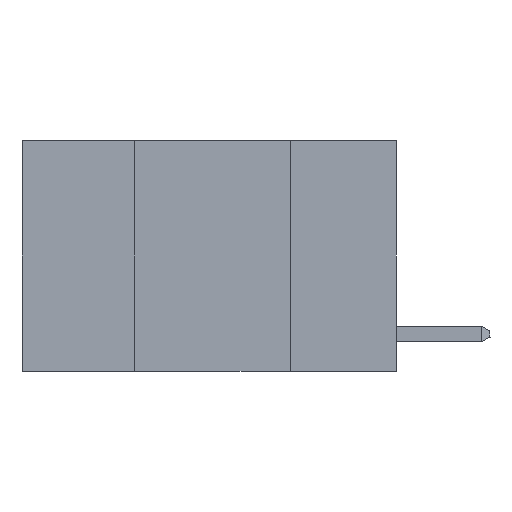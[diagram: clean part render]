
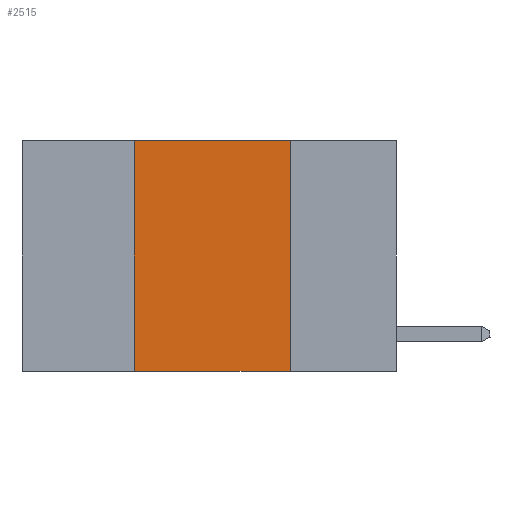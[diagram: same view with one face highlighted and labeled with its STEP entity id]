
A CAD part, left-side view. The second image highlights one B-rep face of the part: STEP entity #2515.
In plain terms, the highlighted planar face has unit normal (-1, 0, 0).
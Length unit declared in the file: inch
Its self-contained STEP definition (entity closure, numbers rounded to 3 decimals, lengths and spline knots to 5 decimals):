
#489 = DIRECTION ( 'NONE',  ( 1., 0., 0. ) ) ;
#502 = DIRECTION ( 'NONE',  ( 0., -1., 0. ) ) ;
#928 = DIRECTION ( 'NONE',  ( 0., 0., 1. ) ) ;
#969 = VECTOR ( 'NONE', #502, 39.37008 ) ;
#1164 = FACE_OUTER_BOUND ( 'NONE', #6510, .T. ) ;
#1691 = ORIENTED_EDGE ( 'NONE', *, *, #2191, .F. ) ;
#2129 = EDGE_CURVE ( 'NONE', #6879, #3749, #4652, .T. ) ;
#2191 = EDGE_CURVE ( 'NONE', #3628, #3103, #7377, .T. ) ;
#2515 = ADVANCED_FACE ( 'NONE', ( #1164 ), #8202, .F. ) ;
#2673 = CARTESIAN_POINT ( 'NONE',  ( 0., 0.17, 0. ) ) ;
#2787 = DIRECTION ( 'NONE',  ( 0., 0., -1. ) ) ;
#2817 = EDGE_CURVE ( 'NONE', #6879, #3628, #7684, .T. ) ;
#2992 = VECTOR ( 'NONE', #928, 39.37008 ) ;
#3103 = VERTEX_POINT ( 'NONE', #6706 ) ;
#3205 = CARTESIAN_POINT ( 'NONE',  ( 0., 0.42, 0. ) ) ;
#3341 = CARTESIAN_POINT ( 'NONE',  ( 0., 0.42, 0. ) ) ;
#3628 = VERTEX_POINT ( 'NONE', #3205 ) ;
#3630 = CARTESIAN_POINT ( 'NONE',  ( 0., 0.17, -0.37 ) ) ;
#3697 = DIRECTION ( 'NONE',  ( 0., -1., 0. ) ) ;
#3749 = VERTEX_POINT ( 'NONE', #3630 ) ;
#3760 = LINE ( 'NONE', #2673, #6738 ) ;
#4336 = ORIENTED_EDGE ( 'NONE', *, *, #2817, .F. ) ;
#4639 = CARTESIAN_POINT ( 'NONE',  ( 0., 0.6, 0. ) ) ;
#4652 = LINE ( 'NONE', #8216, #969 ) ;
#5410 = CARTESIAN_POINT ( 'NONE',  ( 0., 0.42, -0.37 ) ) ;
#5524 = ORIENTED_EDGE ( 'NONE', *, *, #10868, .F. ) ;
#6510 = EDGE_LOOP ( 'NONE', ( #5524, #1691, #4336, #6657 ) ) ;
#6515 = VECTOR ( 'NONE', #3697, 39.37008 ) ;
#6657 = ORIENTED_EDGE ( 'NONE', *, *, #2129, .T. ) ;
#6706 = CARTESIAN_POINT ( 'NONE',  ( 0., 0.17, 0. ) ) ;
#6738 = VECTOR ( 'NONE', #2787, 39.37008 ) ;
#6879 = VERTEX_POINT ( 'NONE', #5410 ) ;
#7377 = LINE ( 'NONE', #10785, #6515 ) ;
#7684 = LINE ( 'NONE', #3341, #2992 ) ;
#8202 = PLANE ( 'NONE',  #8558 ) ;
#8216 = CARTESIAN_POINT ( 'NONE',  ( 0., 0.6, -0.37 ) ) ;
#8558 = AXIS2_PLACEMENT_3D ( 'NONE', #4639, #489, #9872 ) ;
#9872 = DIRECTION ( 'NONE',  ( 0., 0., -1. ) ) ;
#10785 = CARTESIAN_POINT ( 'NONE',  ( 0., 0.6, 0. ) ) ;
#10868 = EDGE_CURVE ( 'NONE', #3103, #3749, #3760, .T. ) ;
